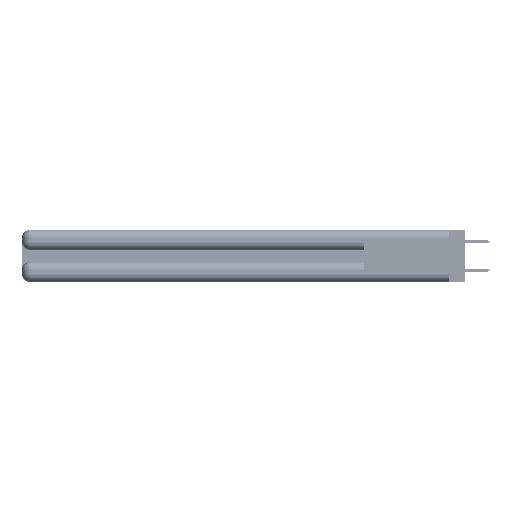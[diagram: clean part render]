
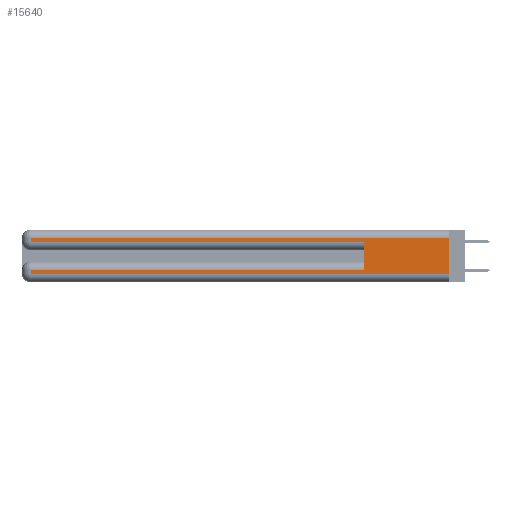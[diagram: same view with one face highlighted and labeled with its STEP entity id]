
A CAD part, left-side view. The second image highlights one B-rep face of the part: STEP entity #15640.
In plain terms, the highlighted planar face has unit normal (-1, 0, 0).
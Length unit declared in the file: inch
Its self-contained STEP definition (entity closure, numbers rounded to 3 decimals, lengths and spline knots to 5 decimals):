
#739 = FACE_OUTER_BOUND ( 'NONE', #50042, .T. ) ;
#2097 = CARTESIAN_POINT ( 'NONE',  ( 0., 0., 0.31 ) ) ;
#2136 = VERTEX_POINT ( 'NONE', #24931 ) ;
#2746 = ORIENTED_EDGE ( 'NONE', *, *, #37945, .F. ) ;
#3021 = DIRECTION ( 'NONE',  ( 0., 0., -1. ) ) ;
#3181 = ORIENTED_EDGE ( 'NONE', *, *, #28394, .T. ) ;
#3373 = VERTEX_POINT ( 'NONE', #17954 ) ;
#3408 = DIRECTION ( 'NONE',  ( 0., 1., 0. ) ) ;
#4871 = CARTESIAN_POINT ( 'NONE',  ( 0., 0., 0.31 ) ) ;
#5448 = VECTOR ( 'NONE', #3021, 39.37008 ) ;
#6832 = CARTESIAN_POINT ( 'NONE',  ( 0., 2.94, 0.085 ) ) ;
#7432 = LINE ( 'NONE', #28278, #48314 ) ;
#7584 = VECTOR ( 'NONE', #18083, 39.37008 ) ;
#8001 = DIRECTION ( 'NONE',  ( 1., 0., 0. ) ) ;
#8832 = VECTOR ( 'NONE', #26039, 39.37008 ) ;
#10562 = CARTESIAN_POINT ( 'NONE',  ( 0., 0., 0.285 ) ) ;
#11877 = VERTEX_POINT ( 'NONE', #16114 ) ;
#12178 = ORIENTED_EDGE ( 'NONE', *, *, #28689, .T. ) ;
#12883 = ORIENTED_EDGE ( 'NONE', *, *, #16827, .T. ) ;
#13235 = LINE ( 'NONE', #22775, #41040 ) ;
#13320 = CARTESIAN_POINT ( 'NONE',  ( 0., 2.94, 0.37 ) ) ;
#13636 = VERTEX_POINT ( 'NONE', #43636 ) ;
#13737 = ORIENTED_EDGE ( 'NONE', *, *, #46851, .T. ) ;
#14165 = VERTEX_POINT ( 'NONE', #6832 ) ;
#15640 = ADVANCED_FACE ( 'NONE', ( #739 ), #31823, .F. ) ;
#16114 = CARTESIAN_POINT ( 'NONE',  ( 0., 0.6, 0.285 ) ) ;
#16196 = AXIS2_PLACEMENT_3D ( 'NONE', #19928, #8001, #35782 ) ;
#16722 = DIRECTION ( 'NONE',  ( 0., 0., 1. ) ) ;
#16827 = EDGE_CURVE ( 'NONE', #14165, #27248, #13235, .T. ) ;
#17101 = VERTEX_POINT ( 'NONE', #4871 ) ;
#17330 = DIRECTION ( 'NONE',  ( 0., 0., -1. ) ) ;
#17954 = CARTESIAN_POINT ( 'NONE',  ( 0., 0.6, 0.085 ) ) ;
#18083 = DIRECTION ( 'NONE',  ( 0., -1., 0. ) ) ;
#18253 = CARTESIAN_POINT ( 'NONE',  ( 0., 2.94, 0.31 ) ) ;
#18258 = LINE ( 'NONE', #2097, #8832 ) ;
#18789 = EDGE_CURVE ( 'NONE', #3373, #11877, #7432, .T. ) ;
#19518 = LINE ( 'NONE', #33824, #7584 ) ;
#19928 = CARTESIAN_POINT ( 'NONE',  ( 0., 0., 0.37 ) ) ;
#22775 = CARTESIAN_POINT ( 'NONE',  ( 0., 2.94, 0.37 ) ) ;
#24931 = CARTESIAN_POINT ( 'NONE',  ( 0., 0., 0.06 ) ) ;
#26039 = DIRECTION ( 'NONE',  ( 0., 1., 0. ) ) ;
#27248 = VERTEX_POINT ( 'NONE', #41372 ) ;
#27934 = LINE ( 'NONE', #30898, #5448 ) ;
#28130 = ORIENTED_EDGE ( 'NONE', *, *, #34674, .T. ) ;
#28278 = CARTESIAN_POINT ( 'NONE',  ( 0., 0.6, 0.145 ) ) ;
#28381 = ORIENTED_EDGE ( 'NONE', *, *, #46838, .T. ) ;
#28394 = EDGE_CURVE ( 'NONE', #46861, #13636, #41975, .T. ) ;
#28689 = EDGE_CURVE ( 'NONE', #3373, #14165, #30897, .T. ) ;
#30691 = DIRECTION ( 'NONE',  ( 0., 0., -1. ) ) ;
#30897 = LINE ( 'NONE', #31281, #40113 ) ;
#30898 = CARTESIAN_POINT ( 'NONE',  ( 0., 0., 0.37 ) ) ;
#31281 = CARTESIAN_POINT ( 'NONE',  ( 0., 0., 0.085 ) ) ;
#31299 = VECTOR ( 'NONE', #34341, 39.37008 ) ;
#31536 = VECTOR ( 'NONE', #17330, 39.37008 ) ;
#31823 = PLANE ( 'NONE',  #16196 ) ;
#33794 = LINE ( 'NONE', #10562, #31299 ) ;
#33824 = CARTESIAN_POINT ( 'NONE',  ( 0., 0., 0.06 ) ) ;
#34341 = DIRECTION ( 'NONE',  ( 0., -1., 0. ) ) ;
#34674 = EDGE_CURVE ( 'NONE', #13636, #11877, #33794, .T. ) ;
#35782 = DIRECTION ( 'NONE',  ( 0., 0., -1. ) ) ;
#37945 = EDGE_CURVE ( 'NONE', #17101, #2136, #27934, .T. ) ;
#40113 = VECTOR ( 'NONE', #3408, 39.37008 ) ;
#41040 = VECTOR ( 'NONE', #30691, 39.37008 ) ;
#41372 = CARTESIAN_POINT ( 'NONE',  ( 0., 2.94, 0.06 ) ) ;
#41975 = LINE ( 'NONE', #13320, #31536 ) ;
#43636 = CARTESIAN_POINT ( 'NONE',  ( 0., 2.94, 0.285 ) ) ;
#43639 = ORIENTED_EDGE ( 'NONE', *, *, #18789, .F. ) ;
#46838 = EDGE_CURVE ( 'NONE', #27248, #2136, #19518, .T. ) ;
#46851 = EDGE_CURVE ( 'NONE', #17101, #46861, #18258, .T. ) ;
#46861 = VERTEX_POINT ( 'NONE', #18253 ) ;
#48314 = VECTOR ( 'NONE', #16722, 39.37008 ) ;
#50042 = EDGE_LOOP ( 'NONE', ( #2746, #13737, #3181, #28130, #43639, #12178, #12883, #28381 ) ) ;
